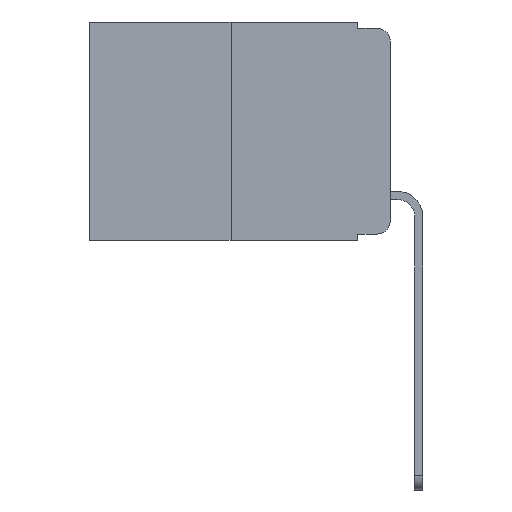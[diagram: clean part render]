
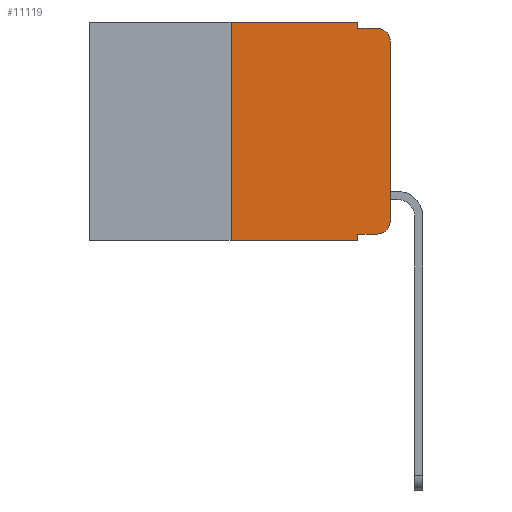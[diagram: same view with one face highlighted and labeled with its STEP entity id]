
A CAD part, left-side view. The second image highlights one B-rep face of the part: STEP entity #11119.
In plain terms, the highlighted planar face has unit normal (-1, 0, 0).
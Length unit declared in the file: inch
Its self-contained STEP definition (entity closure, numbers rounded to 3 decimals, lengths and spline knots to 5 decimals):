
#42 = CARTESIAN_POINT ( 'NONE',  ( 0., 0.02, -0.03 ) ) ;
#346 = VERTEX_POINT ( 'NONE', #6096 ) ;
#378 = VECTOR ( 'NONE', #4019, 39.37008 ) ;
#702 = EDGE_LOOP ( 'NONE', ( #2657, #8669, #746, #12694, #11165, #1428, #7759, #6033, #2542, #12120 ) ) ;
#746 = ORIENTED_EDGE ( 'NONE', *, *, #6448, .F. ) ;
#756 = VERTEX_POINT ( 'NONE', #4682 ) ;
#778 = CARTESIAN_POINT ( 'NONE',  ( 0., 0.25, -0.343 ) ) ;
#811 = CARTESIAN_POINT ( 'NONE',  ( 0., 0.02, -0.313 ) ) ;
#967 = VERTEX_POINT ( 'NONE', #11971 ) ;
#1088 = LINE ( 'NONE', #12586, #3477 ) ;
#1167 = DIRECTION ( 'NONE',  ( 0., 0., -1. ) ) ;
#1171 = VERTEX_POINT ( 'NONE', #9296 ) ;
#1232 = AXIS2_PLACEMENT_3D ( 'NONE', #42, #7237, #1167 ) ;
#1294 = VERTEX_POINT ( 'NONE', #6920 ) ;
#1308 = VECTOR ( 'NONE', #3865, 39.37008 ) ;
#1387 = VERTEX_POINT ( 'NONE', #5864 ) ;
#1428 = ORIENTED_EDGE ( 'NONE', *, *, #5113, .F. ) ;
#1844 = DIRECTION ( 'NONE',  ( 0., 0., -1. ) ) ;
#1900 = DIRECTION ( 'NONE',  ( 0., 0., 1. ) ) ;
#2309 = VERTEX_POINT ( 'NONE', #3515 ) ;
#2452 = VECTOR ( 'NONE', #10672, 39.37008 ) ;
#2542 = ORIENTED_EDGE ( 'NONE', *, *, #3751, .T. ) ;
#2657 = ORIENTED_EDGE ( 'NONE', *, *, #7805, .T. ) ;
#2898 = FACE_OUTER_BOUND ( 'NONE', #702, .T. ) ;
#3076 = EDGE_CURVE ( 'NONE', #346, #1294, #8392, .T. ) ;
#3161 = DIRECTION ( 'NONE',  ( 0., 0., 1. ) ) ;
#3269 = DIRECTION ( 'NONE',  ( 0., 0., -1. ) ) ;
#3477 = VECTOR ( 'NONE', #6640, 39.37008 ) ;
#3515 = CARTESIAN_POINT ( 'NONE',  ( 0., 0.25, 0. ) ) ;
#3751 = EDGE_CURVE ( 'NONE', #967, #346, #1088, .T. ) ;
#3821 = DIRECTION ( 'NONE',  ( 0., -1., 0. ) ) ;
#3865 = DIRECTION ( 'NONE',  ( 0., -1., 0. ) ) ;
#4019 = DIRECTION ( 'NONE',  ( 0., -1., 0. ) ) ;
#4021 = LINE ( 'NONE', #9876, #1308 ) ;
#4439 = EDGE_CURVE ( 'NONE', #967, #12924, #5171, .T. ) ;
#4682 = CARTESIAN_POINT ( 'NONE',  ( 0., 0., -0.03 ) ) ;
#4992 = CARTESIAN_POINT ( 'NONE',  ( 0., 0.473, 0. ) ) ;
#5113 = EDGE_CURVE ( 'NONE', #10026, #2309, #5468, .T. ) ;
#5171 = LINE ( 'NONE', #9675, #2452 ) ;
#5298 = AXIS2_PLACEMENT_3D ( 'NONE', #811, #7917, #1844 ) ;
#5468 = LINE ( 'NONE', #8971, #8135 ) ;
#5779 = EDGE_CURVE ( 'NONE', #1171, #1387, #11661, .T. ) ;
#5827 = LINE ( 'NONE', #4992, #378 ) ;
#5864 = CARTESIAN_POINT ( 'NONE',  ( 0., 0.051, -0.01 ) ) ;
#6033 = ORIENTED_EDGE ( 'NONE', *, *, #4439, .F. ) ;
#6096 = CARTESIAN_POINT ( 'NONE',  ( 0., 0.02, -0.333 ) ) ;
#6448 = EDGE_CURVE ( 'NONE', #1387, #6521, #12720, .T. ) ;
#6521 = VERTEX_POINT ( 'NONE', #10898 ) ;
#6640 = DIRECTION ( 'NONE',  ( 0., -1., 0. ) ) ;
#6920 = CARTESIAN_POINT ( 'NONE',  ( 0., 0., -0.313 ) ) ;
#7133 = EDGE_CURVE ( 'NONE', #756, #6521, #7291, .T. ) ;
#7151 = VECTOR ( 'NONE', #3821, 39.37008 ) ;
#7200 = CARTESIAN_POINT ( 'NONE',  ( 0., 0.051, 0. ) ) ;
#7209 = AXIS2_PLACEMENT_3D ( 'NONE', #9252, #9293, #3269 ) ;
#7237 = DIRECTION ( 'NONE',  ( -1., 0., 0. ) ) ;
#7291 = CIRCLE ( 'NONE', #1232, 0.02 ) ;
#7722 = EDGE_CURVE ( 'NONE', #2309, #1171, #5827, .T. ) ;
#7759 = ORIENTED_EDGE ( 'NONE', *, *, #10878, .T. ) ;
#7805 = EDGE_CURVE ( 'NONE', #1294, #756, #12202, .T. ) ;
#7917 = DIRECTION ( 'NONE',  ( -1., 0., 0. ) ) ;
#8135 = VECTOR ( 'NONE', #1900, 39.37008 ) ;
#8298 = PLANE ( 'NONE',  #7209 ) ;
#8392 = CIRCLE ( 'NONE', #5298, 0.02 ) ;
#8669 = ORIENTED_EDGE ( 'NONE', *, *, #7133, .T. ) ;
#8971 = CARTESIAN_POINT ( 'NONE',  ( 0., 0.25, 0. ) ) ;
#9042 = VECTOR ( 'NONE', #9203, 39.37008 ) ;
#9188 = CARTESIAN_POINT ( 'NONE',  ( 0., 0., 0. ) ) ;
#9203 = DIRECTION ( 'NONE',  ( 0., 0., -1. ) ) ;
#9252 = CARTESIAN_POINT ( 'NONE',  ( 0., 0.473, 0. ) ) ;
#9293 = DIRECTION ( 'NONE',  ( 1., 0., 0. ) ) ;
#9296 = CARTESIAN_POINT ( 'NONE',  ( 0., 0.051, 0. ) ) ;
#9675 = CARTESIAN_POINT ( 'NONE',  ( 0., 0.051, 0. ) ) ;
#9876 = CARTESIAN_POINT ( 'NONE',  ( 0., 0.473, -0.343 ) ) ;
#9894 = VECTOR ( 'NONE', #3161, 39.37008 ) ;
#10026 = VERTEX_POINT ( 'NONE', #778 ) ;
#10672 = DIRECTION ( 'NONE',  ( 0., 0., -1. ) ) ;
#10812 = CARTESIAN_POINT ( 'NONE',  ( 0., 0.051, -0.01 ) ) ;
#10878 = EDGE_CURVE ( 'NONE', #10026, #12924, #4021, .T. ) ;
#10898 = CARTESIAN_POINT ( 'NONE',  ( 0., 0.02, -0.01 ) ) ;
#11119 = ADVANCED_FACE ( 'NONE', ( #2898 ), #8298, .F. ) ;
#11165 = ORIENTED_EDGE ( 'NONE', *, *, #7722, .F. ) ;
#11363 = CARTESIAN_POINT ( 'NONE',  ( 0., 0.051, -0.343 ) ) ;
#11661 = LINE ( 'NONE', #7200, #9042 ) ;
#11971 = CARTESIAN_POINT ( 'NONE',  ( 0., 0.051, -0.333 ) ) ;
#12120 = ORIENTED_EDGE ( 'NONE', *, *, #3076, .T. ) ;
#12202 = LINE ( 'NONE', #9188, #9894 ) ;
#12586 = CARTESIAN_POINT ( 'NONE',  ( 0., 0.051, -0.333 ) ) ;
#12694 = ORIENTED_EDGE ( 'NONE', *, *, #5779, .F. ) ;
#12720 = LINE ( 'NONE', #10812, #7151 ) ;
#12924 = VERTEX_POINT ( 'NONE', #11363 ) ;
